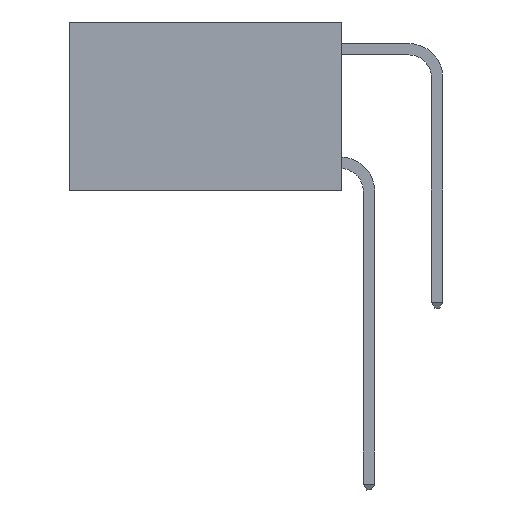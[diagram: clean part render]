
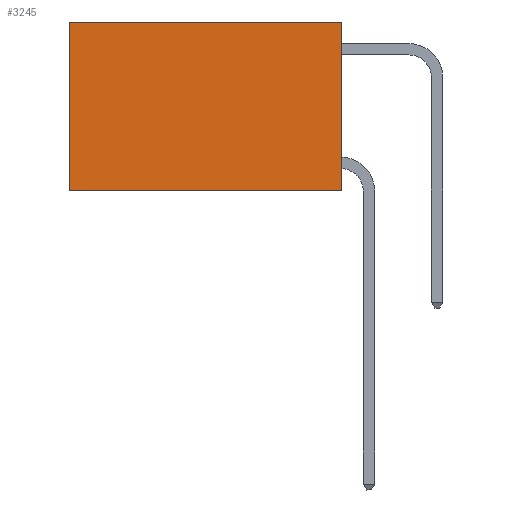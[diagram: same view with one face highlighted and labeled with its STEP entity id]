
A CAD part, left-side view. The second image highlights one B-rep face of the part: STEP entity #3245.
In plain terms, the highlighted planar face has unit normal (-1, 0, 0).
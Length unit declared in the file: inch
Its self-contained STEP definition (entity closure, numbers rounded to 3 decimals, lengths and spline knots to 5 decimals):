
#490 = CARTESIAN_POINT ( 'NONE',  ( 0.2625, 0., 0. ) ) ;
#893 = ORIENTED_EDGE ( 'NONE', *, *, #3530, .F. ) ;
#958 = VECTOR ( 'NONE', #2572, 39.37008 ) ;
#994 = CARTESIAN_POINT ( 'NONE',  ( 0.2625, 0.6, 0. ) ) ;
#1202 = DIRECTION ( 'NONE',  ( 0., 1., 0. ) ) ;
#1213 = VERTEX_POINT ( 'NONE', #2342 ) ;
#1313 = AXIS2_PLACEMENT_3D ( 'NONE', #490, #3833, #5660 ) ;
#1415 = VECTOR ( 'NONE', #4339, 39.37008 ) ;
#1818 = CARTESIAN_POINT ( 'NONE',  ( 0.2625, 0.6, -0.37 ) ) ;
#2115 = FACE_OUTER_BOUND ( 'NONE', #6411, .T. ) ;
#2342 = CARTESIAN_POINT ( 'NONE',  ( 0.2625, 0., 0. ) ) ;
#2451 = VERTEX_POINT ( 'NONE', #10533 ) ;
#2458 = CARTESIAN_POINT ( 'NONE',  ( 0.2625, 0., -0.37 ) ) ;
#2572 = DIRECTION ( 'NONE',  ( 0., 1., 0. ) ) ;
#3068 = PLANE ( 'NONE',  #1313 ) ;
#3245 = ADVANCED_FACE ( 'NONE', ( #2115 ), #3068, .F. ) ;
#3530 = EDGE_CURVE ( 'NONE', #1213, #2451, #6894, .T. ) ;
#3676 = CARTESIAN_POINT ( 'NONE',  ( 0.2625, 0., 0. ) ) ;
#3833 = DIRECTION ( 'NONE',  ( 1., 0., 0. ) ) ;
#4339 = DIRECTION ( 'NONE',  ( 0., 0., -1. ) ) ;
#4406 = EDGE_CURVE ( 'NONE', #8850, #10705, #8515, .T. ) ;
#4480 = VECTOR ( 'NONE', #10269, 39.37008 ) ;
#5660 = DIRECTION ( 'NONE',  ( 0., 0., -1. ) ) ;
#6259 = EDGE_CURVE ( 'NONE', #1213, #8850, #8023, .T. ) ;
#6411 = EDGE_LOOP ( 'NONE', ( #7505, #6707, #893, #10011 ) ) ;
#6705 = VECTOR ( 'NONE', #1202, 39.37008 ) ;
#6707 = ORIENTED_EDGE ( 'NONE', *, *, #10267, .F. ) ;
#6894 = LINE ( 'NONE', #10155, #4480 ) ;
#7505 = ORIENTED_EDGE ( 'NONE', *, *, #4406, .T. ) ;
#8023 = LINE ( 'NONE', #3676, #6705 ) ;
#8515 = LINE ( 'NONE', #994, #1415 ) ;
#8850 = VERTEX_POINT ( 'NONE', #10524 ) ;
#9985 = LINE ( 'NONE', #2458, #958 ) ;
#10011 = ORIENTED_EDGE ( 'NONE', *, *, #6259, .T. ) ;
#10155 = CARTESIAN_POINT ( 'NONE',  ( 0.2625, 0., 0. ) ) ;
#10267 = EDGE_CURVE ( 'NONE', #2451, #10705, #9985, .T. ) ;
#10269 = DIRECTION ( 'NONE',  ( 0., 0., -1. ) ) ;
#10524 = CARTESIAN_POINT ( 'NONE',  ( 0.2625, 0.6, 0. ) ) ;
#10533 = CARTESIAN_POINT ( 'NONE',  ( 0.2625, 0., -0.37 ) ) ;
#10705 = VERTEX_POINT ( 'NONE', #1818 ) ;
